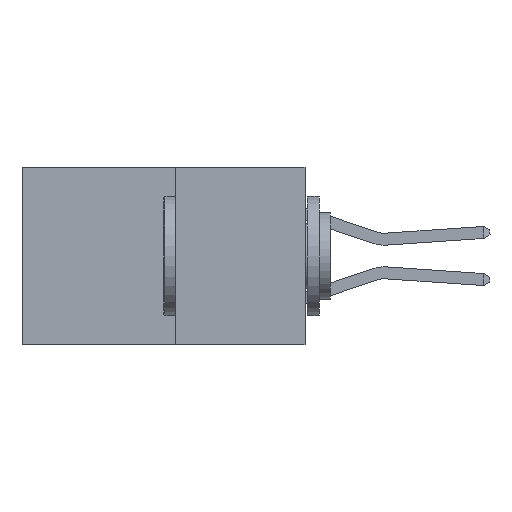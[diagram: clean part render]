
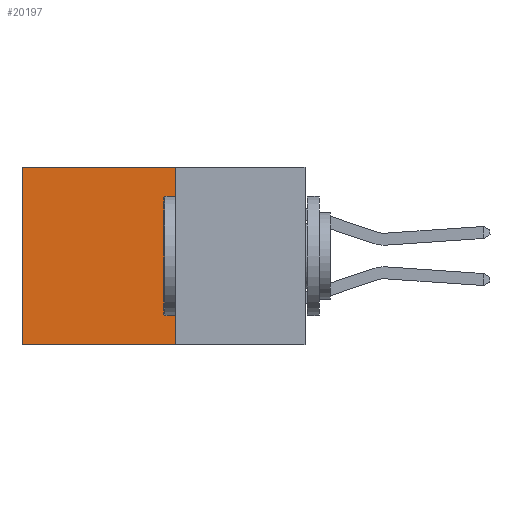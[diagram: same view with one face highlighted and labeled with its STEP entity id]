
A CAD part, left-side view. The second image highlights one B-rep face of the part: STEP entity #20197.
In plain terms, the highlighted planar face has unit normal (-1, 0, 0).
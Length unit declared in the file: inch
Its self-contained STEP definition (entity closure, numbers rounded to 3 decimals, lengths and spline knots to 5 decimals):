
#1197 = DIRECTION ( 'NONE',  ( 0., 0., -1. ) ) ;
#2223 = ORIENTED_EDGE ( 'NONE', *, *, #3408, .F. ) ;
#2887 = ORIENTED_EDGE ( 'NONE', *, *, #14813, .T. ) ;
#3408 = EDGE_CURVE ( 'NONE', #11724, #16130, #7728, .T. ) ;
#3903 = VERTEX_POINT ( 'NONE', #28789 ) ;
#4405 = CARTESIAN_POINT ( 'NONE',  ( 0.277, 0.27, 0. ) ) ;
#7001 = VECTOR ( 'NONE', #11920, 39.37008 ) ;
#7728 = LINE ( 'NONE', #13567, #25693 ) ;
#7744 = DIRECTION ( 'NONE',  ( 0., 1., 0. ) ) ;
#8886 = VECTOR ( 'NONE', #1197, 39.37008 ) ;
#9394 = CARTESIAN_POINT ( 'NONE',  ( 0.277, 0.27, -0.37 ) ) ;
#10256 = LINE ( 'NONE', #26457, #15742 ) ;
#11364 = DIRECTION ( 'NONE',  ( 0., 0., -1. ) ) ;
#11724 = VERTEX_POINT ( 'NONE', #4405 ) ;
#11920 = DIRECTION ( 'NONE',  ( 0., 1., 0. ) ) ;
#12683 = CARTESIAN_POINT ( 'NONE',  ( 0.277, 0.59, 0. ) ) ;
#13083 = DIRECTION ( 'NONE',  ( 0., 0., -1. ) ) ;
#13567 = CARTESIAN_POINT ( 'NONE',  ( 0.277, 0.27, -0.37 ) ) ;
#14813 = EDGE_CURVE ( 'NONE', #26505, #3903, #16562, .T. ) ;
#15590 = AXIS2_PLACEMENT_3D ( 'NONE', #27515, #25424, #11364 ) ;
#15742 = VECTOR ( 'NONE', #7744, 39.37008 ) ;
#16130 = VERTEX_POINT ( 'NONE', #9394 ) ;
#16562 = LINE ( 'NONE', #19930, #8886 ) ;
#18371 = ORIENTED_EDGE ( 'NONE', *, *, #26961, .F. ) ;
#19930 = CARTESIAN_POINT ( 'NONE',  ( 0.277, 0.59, -0.37 ) ) ;
#20197 = ADVANCED_FACE ( 'NONE', ( #20997 ), #29938, .F. ) ;
#20997 = FACE_OUTER_BOUND ( 'NONE', #25186, .T. ) ;
#21271 = CARTESIAN_POINT ( 'NONE',  ( 0.277, 0.27, -0.37 ) ) ;
#21774 = ORIENTED_EDGE ( 'NONE', *, *, #27101, .T. ) ;
#25186 = EDGE_LOOP ( 'NONE', ( #2887, #18371, #2223, #21774 ) ) ;
#25424 = DIRECTION ( 'NONE',  ( 1., 0., 0. ) ) ;
#25678 = LINE ( 'NONE', #21271, #7001 ) ;
#25693 = VECTOR ( 'NONE', #13083, 39.37008 ) ;
#26457 = CARTESIAN_POINT ( 'NONE',  ( 0.277, 0.27, 0. ) ) ;
#26505 = VERTEX_POINT ( 'NONE', #12683 ) ;
#26961 = EDGE_CURVE ( 'NONE', #16130, #3903, #25678, .T. ) ;
#27101 = EDGE_CURVE ( 'NONE', #11724, #26505, #10256, .T. ) ;
#27515 = CARTESIAN_POINT ( 'NONE',  ( 0.277, 0.27, -0.37 ) ) ;
#28789 = CARTESIAN_POINT ( 'NONE',  ( 0.277, 0.59, -0.37 ) ) ;
#29938 = PLANE ( 'NONE',  #15590 ) ;
